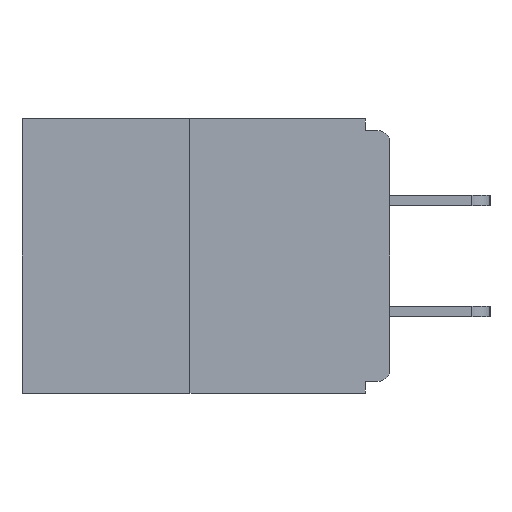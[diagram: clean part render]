
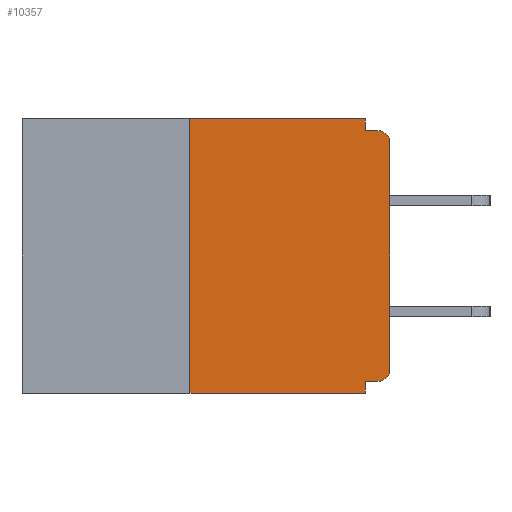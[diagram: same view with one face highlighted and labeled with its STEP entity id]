
A CAD part, left-side view. The second image highlights one B-rep face of the part: STEP entity #10357.
In plain terms, the highlighted planar face has unit normal (-1, 0, 0).
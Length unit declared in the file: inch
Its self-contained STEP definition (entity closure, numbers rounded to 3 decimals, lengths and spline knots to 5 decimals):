
#104 = VERTEX_POINT ( 'NONE', #10232 ) ;
#338 = FACE_OUTER_BOUND ( 'NONE', #9476, .T. ) ;
#555 = DIRECTION ( 'NONE',  ( 0., 0., 1. ) ) ;
#695 = DIRECTION ( 'NONE',  ( 0., 0., -1. ) ) ;
#1152 = VECTOR ( 'NONE', #555, 39.37008 ) ;
#1241 = DIRECTION ( 'NONE',  ( 0., -1., 0. ) ) ;
#1299 = ORIENTED_EDGE ( 'NONE', *, *, #8876, .T. ) ;
#1338 = AXIS2_PLACEMENT_3D ( 'NONE', #9487, #3102, #11451 ) ;
#1452 = VERTEX_POINT ( 'NONE', #12859 ) ;
#1491 = ORIENTED_EDGE ( 'NONE', *, *, #12514, .F. ) ;
#1696 = ORIENTED_EDGE ( 'NONE', *, *, #10124, .F. ) ;
#1796 = CARTESIAN_POINT ( 'NONE',  ( 0., 0.46, 0. ) ) ;
#1841 = DIRECTION ( 'NONE',  ( 0., 1., 0. ) ) ;
#2172 = VERTEX_POINT ( 'NONE', #16534 ) ;
#2221 = CARTESIAN_POINT ( 'NONE',  ( 0., 0.015, -0.328 ) ) ;
#2402 = VERTEX_POINT ( 'NONE', #2221 ) ;
#2624 = VERTEX_POINT ( 'NONE', #14122 ) ;
#2725 = DIRECTION ( 'NONE',  ( 0., 0., 1. ) ) ;
#3102 = DIRECTION ( 'NONE',  ( -1., 0., 0. ) ) ;
#3129 = LINE ( 'NONE', #7399, #14950 ) ;
#3349 = LINE ( 'NONE', #13030, #9207 ) ;
#3427 = EDGE_CURVE ( 'NONE', #2402, #2624, #14518, .T. ) ;
#3647 = VECTOR ( 'NONE', #8798, 39.37008 ) ;
#4033 = ORIENTED_EDGE ( 'NONE', *, *, #14026, .F. ) ;
#5298 = VERTEX_POINT ( 'NONE', #7823 ) ;
#5884 = PLANE ( 'NONE',  #7994 ) ;
#5934 = VERTEX_POINT ( 'NONE', #10951 ) ;
#6134 = EDGE_CURVE ( 'NONE', #1452, #10980, #11550, .T. ) ;
#6135 = CARTESIAN_POINT ( 'NONE',  ( 0., 0., -0.03 ) ) ;
#6146 = VERTEX_POINT ( 'NONE', #8938 ) ;
#7075 = EDGE_CURVE ( 'NONE', #2172, #5934, #17750, .T. ) ;
#7257 = EDGE_CURVE ( 'NONE', #10980, #5298, #12775, .T. ) ;
#7399 = CARTESIAN_POINT ( 'NONE',  ( 0., 0.46, 0. ) ) ;
#7823 = CARTESIAN_POINT ( 'NONE',  ( 0., 0.015, -0.015 ) ) ;
#7927 = CARTESIAN_POINT ( 'NONE',  ( 0., 0.46, -0.343 ) ) ;
#7994 = AXIS2_PLACEMENT_3D ( 'NONE', #1796, #16932, #9797 ) ;
#8179 = ORIENTED_EDGE ( 'NONE', *, *, #3427, .F. ) ;
#8184 = AXIS2_PLACEMENT_3D ( 'NONE', #13123, #15739, #695 ) ;
#8798 = DIRECTION ( 'NONE',  ( 0., 0., -1. ) ) ;
#8876 = EDGE_CURVE ( 'NONE', #6146, #10281, #9269, .T. ) ;
#8938 = CARTESIAN_POINT ( 'NONE',  ( 0., 0.25, -0.343 ) ) ;
#9207 = VECTOR ( 'NONE', #10418, 39.37008 ) ;
#9269 = LINE ( 'NONE', #7927, #15714 ) ;
#9476 = EDGE_LOOP ( 'NONE', ( #1491, #1696, #1299, #10192, #8179, #17558, #17454, #13120, #4033, #11870 ) ) ;
#9487 = CARTESIAN_POINT ( 'NONE',  ( 0., 0.015, -0.313 ) ) ;
#9797 = DIRECTION ( 'NONE',  ( 0., 0., -1. ) ) ;
#10124 = EDGE_CURVE ( 'NONE', #6146, #104, #12155, .T. ) ;
#10188 = CARTESIAN_POINT ( 'NONE',  ( 0., 0., 0. ) ) ;
#10192 = ORIENTED_EDGE ( 'NONE', *, *, #10801, .F. ) ;
#10232 = CARTESIAN_POINT ( 'NONE',  ( 0., 0.25, 0. ) ) ;
#10281 = VERTEX_POINT ( 'NONE', #15379 ) ;
#10357 = ADVANCED_FACE ( 'NONE', ( #338 ), #5884, .F. ) ;
#10418 = DIRECTION ( 'NONE',  ( 0., -1., 0. ) ) ;
#10801 = EDGE_CURVE ( 'NONE', #2624, #10281, #12576, .T. ) ;
#10886 = DIRECTION ( 'NONE',  ( 0., 0., -1. ) ) ;
#10951 = CARTESIAN_POINT ( 'NONE',  ( 0., 0.031, -0.015 ) ) ;
#10980 = VERTEX_POINT ( 'NONE', #6135 ) ;
#11451 = DIRECTION ( 'NONE',  ( 0., 0., -1. ) ) ;
#11550 = LINE ( 'NONE', #10188, #1152 ) ;
#11870 = ORIENTED_EDGE ( 'NONE', *, *, #7075, .F. ) ;
#12155 = LINE ( 'NONE', #14852, #13149 ) ;
#12514 = EDGE_CURVE ( 'NONE', #104, #2172, #3129, .T. ) ;
#12576 = LINE ( 'NONE', #12838, #3647 ) ;
#12775 = CIRCLE ( 'NONE', #8184, 0.015 ) ;
#12838 = CARTESIAN_POINT ( 'NONE',  ( 0., 0.031, -0.343 ) ) ;
#12859 = CARTESIAN_POINT ( 'NONE',  ( 0., 0., -0.313 ) ) ;
#13030 = CARTESIAN_POINT ( 'NONE',  ( 0., 0., -0.015 ) ) ;
#13120 = ORIENTED_EDGE ( 'NONE', *, *, #7257, .T. ) ;
#13123 = CARTESIAN_POINT ( 'NONE',  ( 0., 0.015, -0.03 ) ) ;
#13149 = VECTOR ( 'NONE', #2725, 39.37008 ) ;
#13164 = EDGE_CURVE ( 'NONE', #2402, #1452, #14644, .T. ) ;
#14026 = EDGE_CURVE ( 'NONE', #5934, #5298, #3349, .T. ) ;
#14122 = CARTESIAN_POINT ( 'NONE',  ( 0., 0.031, -0.328 ) ) ;
#14518 = LINE ( 'NONE', #17156, #16872 ) ;
#14644 = CIRCLE ( 'NONE', #1338, 0.015 ) ;
#14852 = CARTESIAN_POINT ( 'NONE',  ( 0., 0.25, 0. ) ) ;
#14950 = VECTOR ( 'NONE', #15605, 39.37008 ) ;
#15358 = VECTOR ( 'NONE', #10886, 39.37008 ) ;
#15379 = CARTESIAN_POINT ( 'NONE',  ( 0., 0.031, -0.343 ) ) ;
#15605 = DIRECTION ( 'NONE',  ( 0., -1., 0. ) ) ;
#15714 = VECTOR ( 'NONE', #1241, 39.37008 ) ;
#15739 = DIRECTION ( 'NONE',  ( -1., 0., 0. ) ) ;
#16534 = CARTESIAN_POINT ( 'NONE',  ( 0., 0.031, 0. ) ) ;
#16872 = VECTOR ( 'NONE', #1841, 39.37008 ) ;
#16932 = DIRECTION ( 'NONE',  ( 1., 0., 0. ) ) ;
#17156 = CARTESIAN_POINT ( 'NONE',  ( 0., 0., -0.328 ) ) ;
#17454 = ORIENTED_EDGE ( 'NONE', *, *, #6134, .T. ) ;
#17558 = ORIENTED_EDGE ( 'NONE', *, *, #13164, .T. ) ;
#17662 = CARTESIAN_POINT ( 'NONE',  ( 0., 0.031, 0. ) ) ;
#17750 = LINE ( 'NONE', #17662, #15358 ) ;
